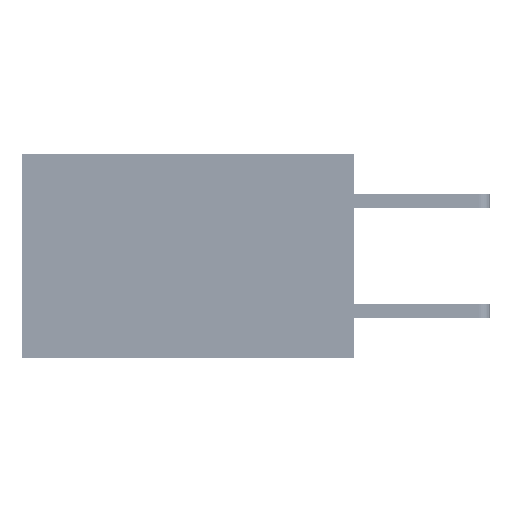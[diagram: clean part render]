
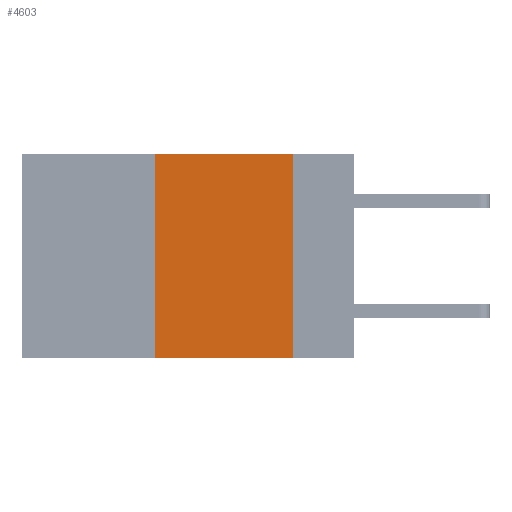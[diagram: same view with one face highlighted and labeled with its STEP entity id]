
A CAD part, left-side view. The second image highlights one B-rep face of the part: STEP entity #4603.
In plain terms, the highlighted planar face has unit normal (-1, 0, 0).
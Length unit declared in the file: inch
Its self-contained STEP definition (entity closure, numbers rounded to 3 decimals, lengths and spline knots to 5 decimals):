
#4603 = ADVANCED_FACE ( 'NONE', ( #19872 ), #34072, .F. ) ;
#5273 = ORIENTED_EDGE ( 'NONE', *, *, #34744, .T. ) ;
#7515 = ORIENTED_EDGE ( 'NONE', *, *, #24729, .F. ) ;
#8173 = ORIENTED_EDGE ( 'NONE', *, *, #16058, .F. ) ;
#9146 = EDGE_LOOP ( 'NONE', ( #8173, #7515, #16302, #5273 ) ) ;
#11232 = CARTESIAN_POINT ( 'NONE',  ( 0., 0.11, 0. ) ) ;
#12825 = EDGE_CURVE ( 'NONE', #33078, #19218, #33446, .T. ) ;
#12832 = LINE ( 'NONE', #23405, #25717 ) ;
#13302 = VERTEX_POINT ( 'NONE', #27683 ) ;
#14093 = DIRECTION ( 'NONE',  ( 0., -1., 0. ) ) ;
#16058 = EDGE_CURVE ( 'NONE', #24820, #13302, #38004, .T. ) ;
#16302 = ORIENTED_EDGE ( 'NONE', *, *, #12825, .F. ) ;
#16533 = CARTESIAN_POINT ( 'NONE',  ( 0., 0.36, 0. ) ) ;
#17969 = VECTOR ( 'NONE', #29709, 39.37008 ) ;
#19218 = VERTEX_POINT ( 'NONE', #16533 ) ;
#19256 = DIRECTION ( 'NONE',  ( 0., 0., -1. ) ) ;
#19872 = FACE_OUTER_BOUND ( 'NONE', #9146, .T. ) ;
#20438 = DIRECTION ( 'NONE',  ( 0., 0., -1. ) ) ;
#23405 = CARTESIAN_POINT ( 'NONE',  ( 0., 0.6, 0. ) ) ;
#23721 = AXIS2_PLACEMENT_3D ( 'NONE', #31556, #28207, #19256 ) ;
#24121 = CARTESIAN_POINT ( 'NONE',  ( 0., 0.36, -0.37 ) ) ;
#24729 = EDGE_CURVE ( 'NONE', #19218, #24820, #12832, .T. ) ;
#24820 = VERTEX_POINT ( 'NONE', #38770 ) ;
#25717 = VECTOR ( 'NONE', #14093, 39.37008 ) ;
#27683 = CARTESIAN_POINT ( 'NONE',  ( 0., 0.11, -0.37 ) ) ;
#28207 = DIRECTION ( 'NONE',  ( 1., 0., 0. ) ) ;
#28218 = VECTOR ( 'NONE', #28544, 39.37008 ) ;
#28544 = DIRECTION ( 'NONE',  ( 0., 0., 1. ) ) ;
#29709 = DIRECTION ( 'NONE',  ( 0., -1., 0. ) ) ;
#29899 = VECTOR ( 'NONE', #20438, 39.37008 ) ;
#31556 = CARTESIAN_POINT ( 'NONE',  ( 0., 0.6, 0. ) ) ;
#33078 = VERTEX_POINT ( 'NONE', #24121 ) ;
#33446 = LINE ( 'NONE', #34270, #28218 ) ;
#34072 = PLANE ( 'NONE',  #23721 ) ;
#34270 = CARTESIAN_POINT ( 'NONE',  ( 0., 0.36, 0. ) ) ;
#34744 = EDGE_CURVE ( 'NONE', #33078, #13302, #39444, .T. ) ;
#38004 = LINE ( 'NONE', #11232, #29899 ) ;
#38239 = CARTESIAN_POINT ( 'NONE',  ( 0., 0.6, -0.37 ) ) ;
#38770 = CARTESIAN_POINT ( 'NONE',  ( 0., 0.11, 0. ) ) ;
#39444 = LINE ( 'NONE', #38239, #17969 ) ;
